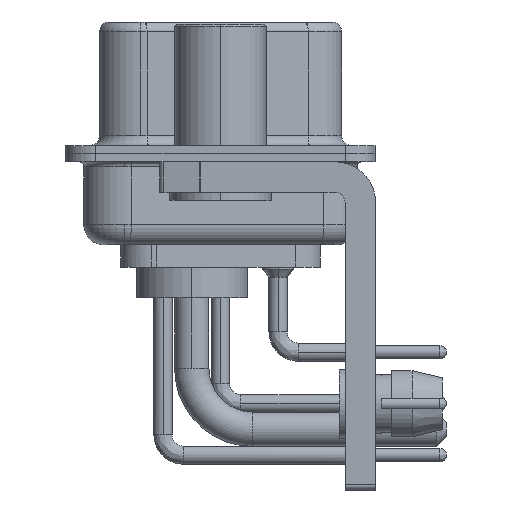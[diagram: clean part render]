
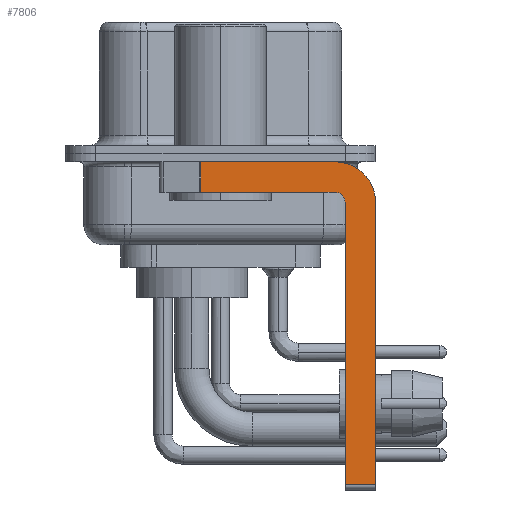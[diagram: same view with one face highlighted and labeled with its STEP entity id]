
A CAD part, left-side view. The second image highlights one B-rep face of the part: STEP entity #7806.
In plain terms, the highlighted planar face has unit normal (-1, 0, 0).
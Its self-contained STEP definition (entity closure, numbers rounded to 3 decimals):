
#10 = LINE ( 'NONE', #11690, #33904 ) ;
#69 = AXIS2_PLACEMENT_3D ( 'NONE', #15274, #15473, #9716 ) ;
#588 = AXIS2_PLACEMENT_3D ( 'NONE', #14721, #23097, #14913 ) ;
#1620 = LINE ( 'NONE', #25290, #35715 ) ;
#2580 = CARTESIAN_POINT ( 'NONE',  ( -2.9, -5.65, -1.9 ) ) ;
#2746 = VECTOR ( 'NONE', #11584, 1000. ) ;
#2884 = LINE ( 'NONE', #14591, #26528 ) ;
#4871 = EDGE_LOOP ( 'NONE', ( #14509, #27020, #12388, #19574, #19040, #25799, #28749, #35435 ) ) ;
#5282 = VERTEX_POINT ( 'NONE', #26368 ) ;
#5366 = DIRECTION ( 'NONE',  ( 0., 0., -1. ) ) ;
#5692 = PLANE ( 'NONE',  #588 ) ;
#7806 = ADVANCED_FACE ( 'NONE', ( #17781 ), #5692, .F. ) ;
#9555 = CARTESIAN_POINT ( 'NONE',  ( -2.9, -7.65, -16.35 ) ) ;
#9716 = DIRECTION ( 'NONE',  ( 0., 0., 1. ) ) ;
#10546 = CIRCLE ( 'NONE', #21567, 2. ) ;
#11584 = DIRECTION ( 'NONE',  ( 0., 1., 0. ) ) ;
#11675 = EDGE_CURVE ( 'NONE', #20405, #17357, #27312, .T. ) ;
#11690 = CARTESIAN_POINT ( 'NONE',  ( -2.9, -5.65, -16.35 ) ) ;
#12388 = ORIENTED_EDGE ( 'NONE', *, *, #34398, .F. ) ;
#12670 = CARTESIAN_POINT ( 'NONE',  ( -2.9, -5.65, -2.4 ) ) ;
#12838 = CARTESIAN_POINT ( 'NONE',  ( -2.9, 3., -0.4 ) ) ;
#13361 = CARTESIAN_POINT ( 'NONE',  ( -2.9, -6.15, -16.35 ) ) ;
#14509 = ORIENTED_EDGE ( 'NONE', *, *, #11675, .F. ) ;
#14591 = CARTESIAN_POINT ( 'NONE',  ( -2.9, -7.65, -2.4 ) ) ;
#14721 = CARTESIAN_POINT ( 'NONE',  ( -2.9, -5.65, -2.4 ) ) ;
#14913 = DIRECTION ( 'NONE',  ( 0., 0., -1. ) ) ;
#14966 = DIRECTION ( 'NONE',  ( 1., 0., 0. ) ) ;
#15274 = CARTESIAN_POINT ( 'NONE',  ( -2.9, -5.65, -2.4 ) ) ;
#15367 = CIRCLE ( 'NONE', #69, 0.5 ) ;
#15473 = DIRECTION ( 'NONE',  ( -1., 0., 0. ) ) ;
#16175 = DIRECTION ( 'NONE',  ( 0., 0., 1. ) ) ;
#17357 = VERTEX_POINT ( 'NONE', #32588 ) ;
#17781 = FACE_OUTER_BOUND ( 'NONE', #4871, .T. ) ;
#19040 = ORIENTED_EDGE ( 'NONE', *, *, #34636, .F. ) ;
#19574 = ORIENTED_EDGE ( 'NONE', *, *, #22469, .F. ) ;
#20405 = VERTEX_POINT ( 'NONE', #21404 ) ;
#20869 = VERTEX_POINT ( 'NONE', #29715 ) ;
#21404 = CARTESIAN_POINT ( 'NONE',  ( -2.9, 0.978, -0.4 ) ) ;
#21479 = VERTEX_POINT ( 'NONE', #9555 ) ;
#21567 = AXIS2_PLACEMENT_3D ( 'NONE', #12670, #14966, #35744 ) ;
#22469 = EDGE_CURVE ( 'NONE', #28569, #20869, #15367, .T. ) ;
#22645 = VERTEX_POINT ( 'NONE', #13361 ) ;
#23097 = DIRECTION ( 'NONE',  ( 1., 0., 0. ) ) ;
#24229 = EDGE_CURVE ( 'NONE', #17357, #33598, #10546, .T. ) ;
#25290 = CARTESIAN_POINT ( 'NONE',  ( -2.9, -6.15, -16.6 ) ) ;
#25588 = EDGE_CURVE ( 'NONE', #33598, #21479, #2884, .T. ) ;
#25624 = LINE ( 'NONE', #31514, #31520 ) ;
#25799 = ORIENTED_EDGE ( 'NONE', *, *, #35386, .T. ) ;
#26368 = CARTESIAN_POINT ( 'NONE',  ( -2.9, 0.978, -1.9 ) ) ;
#26528 = VECTOR ( 'NONE', #34217, 1000. ) ;
#27020 = ORIENTED_EDGE ( 'NONE', *, *, #36769, .T. ) ;
#27312 = LINE ( 'NONE', #12838, #31302 ) ;
#28569 = VERTEX_POINT ( 'NONE', #32927 ) ;
#28749 = ORIENTED_EDGE ( 'NONE', *, *, #25588, .F. ) ;
#29715 = CARTESIAN_POINT ( 'NONE',  ( -2.9, -5.65, -1.9 ) ) ;
#31302 = VECTOR ( 'NONE', #36644, 1000. ) ;
#31499 = CARTESIAN_POINT ( 'NONE',  ( -2.9, -7.65, -2.4 ) ) ;
#31514 = CARTESIAN_POINT ( 'NONE',  ( -2.9, 0.978, -1.9 ) ) ;
#31520 = VECTOR ( 'NONE', #5366, 1000. ) ;
#32178 = LINE ( 'NONE', #2580, #2746 ) ;
#32588 = CARTESIAN_POINT ( 'NONE',  ( -2.9, -5.65, -0.4 ) ) ;
#32927 = CARTESIAN_POINT ( 'NONE',  ( -2.9, -6.15, -2.4 ) ) ;
#33598 = VERTEX_POINT ( 'NONE', #31499 ) ;
#33904 = VECTOR ( 'NONE', #34972, 1000. ) ;
#34217 = DIRECTION ( 'NONE',  ( 0., 0., -1. ) ) ;
#34398 = EDGE_CURVE ( 'NONE', #20869, #5282, #32178, .T. ) ;
#34636 = EDGE_CURVE ( 'NONE', #22645, #28569, #1620, .T. ) ;
#34972 = DIRECTION ( 'NONE',  ( 0., -1., 0. ) ) ;
#35386 = EDGE_CURVE ( 'NONE', #22645, #21479, #10, .T. ) ;
#35435 = ORIENTED_EDGE ( 'NONE', *, *, #24229, .F. ) ;
#35715 = VECTOR ( 'NONE', #16175, 1000. ) ;
#35744 = DIRECTION ( 'NONE',  ( 0., 0., -1. ) ) ;
#36644 = DIRECTION ( 'NONE',  ( 0., -1., 0. ) ) ;
#36769 = EDGE_CURVE ( 'NONE', #20405, #5282, #25624, .T. ) ;
